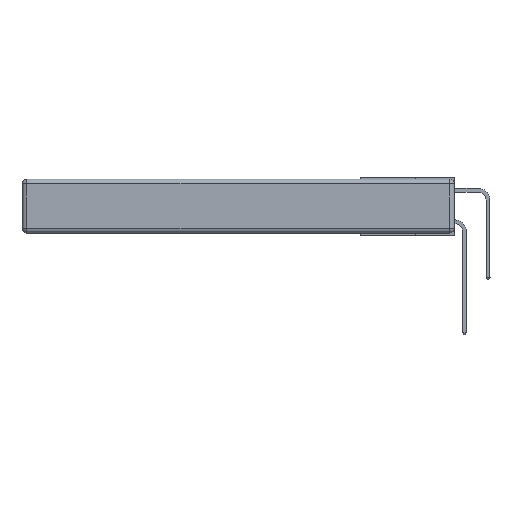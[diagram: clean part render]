
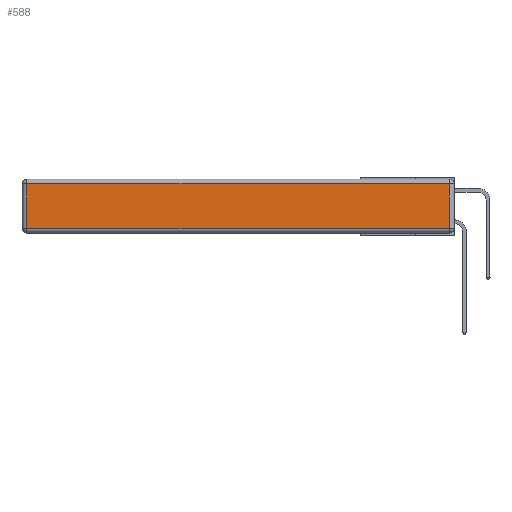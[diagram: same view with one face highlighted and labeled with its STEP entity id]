
A CAD part, left-side view. The second image highlights one B-rep face of the part: STEP entity #588.
In plain terms, the highlighted planar face has unit normal (-1, 0, 0).
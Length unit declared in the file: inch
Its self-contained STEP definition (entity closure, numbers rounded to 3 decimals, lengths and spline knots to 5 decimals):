
#135 = CARTESIAN_POINT ( 'NONE',  ( 0., 0., -0.313 ) ) ;
#588 = ADVANCED_FACE ( 'NONE', ( #12810 ), #10628, .T. ) ;
#835 = LINE ( 'NONE', #135, #6028 ) ;
#850 = VECTOR ( 'NONE', #2423, 39.37008 ) ;
#1299 = VECTOR ( 'NONE', #5944, 39.37008 ) ;
#2312 = DIRECTION ( 'NONE',  ( 0., -1., 0. ) ) ;
#2313 = VECTOR ( 'NONE', #10353, 39.37008 ) ;
#2423 = DIRECTION ( 'NONE',  ( 0., 0., 1. ) ) ;
#2646 = LINE ( 'NONE', #6118, #2313 ) ;
#2875 = VERTEX_POINT ( 'NONE', #3873 ) ;
#2884 = LINE ( 'NONE', #11077, #850 ) ;
#3011 = DIRECTION ( 'NONE',  ( 0., 0., 1. ) ) ;
#3873 = CARTESIAN_POINT ( 'NONE',  ( 0., 0.03, -0.313 ) ) ;
#4459 = CARTESIAN_POINT ( 'NONE',  ( 0., 0.03, -0.03 ) ) ;
#5346 = CARTESIAN_POINT ( 'NONE',  ( 0., 2.72, -0.03 ) ) ;
#5892 = EDGE_LOOP ( 'NONE', ( #9965, #8094, #12895, #7971 ) ) ;
#5944 = DIRECTION ( 'NONE',  ( 0., 1., 0. ) ) ;
#6028 = VECTOR ( 'NONE', #2312, 39.37008 ) ;
#6118 = CARTESIAN_POINT ( 'NONE',  ( 0., 2.72, -0.343 ) ) ;
#7374 = EDGE_CURVE ( 'NONE', #7587, #12016, #8336, .T. ) ;
#7394 = EDGE_CURVE ( 'NONE', #12016, #9848, #2646, .T. ) ;
#7587 = VERTEX_POINT ( 'NONE', #4459 ) ;
#7971 = ORIENTED_EDGE ( 'NONE', *, *, #7394, .T. ) ;
#8094 = ORIENTED_EDGE ( 'NONE', *, *, #10301, .T. ) ;
#8283 = AXIS2_PLACEMENT_3D ( 'NONE', #10542, #12761, #3011 ) ;
#8336 = LINE ( 'NONE', #11329, #1299 ) ;
#9848 = VERTEX_POINT ( 'NONE', #12305 ) ;
#9965 = ORIENTED_EDGE ( 'NONE', *, *, #11079, .T. ) ;
#10301 = EDGE_CURVE ( 'NONE', #2875, #7587, #2884, .T. ) ;
#10353 = DIRECTION ( 'NONE',  ( 0., 0., -1. ) ) ;
#10542 = CARTESIAN_POINT ( 'NONE',  ( 0., 0., -0.343 ) ) ;
#10628 = PLANE ( 'NONE',  #8283 ) ;
#11077 = CARTESIAN_POINT ( 'NONE',  ( 0., 0.03, -0.343 ) ) ;
#11079 = EDGE_CURVE ( 'NONE', #9848, #2875, #835, .T. ) ;
#11329 = CARTESIAN_POINT ( 'NONE',  ( 0., 2.75, -0.03 ) ) ;
#12016 = VERTEX_POINT ( 'NONE', #5346 ) ;
#12305 = CARTESIAN_POINT ( 'NONE',  ( 0., 2.72, -0.313 ) ) ;
#12761 = DIRECTION ( 'NONE',  ( -1., 0., 0. ) ) ;
#12810 = FACE_OUTER_BOUND ( 'NONE', #5892, .T. ) ;
#12895 = ORIENTED_EDGE ( 'NONE', *, *, #7374, .T. ) ;
